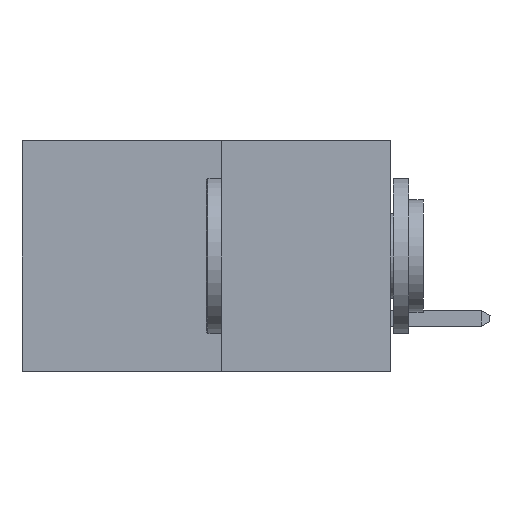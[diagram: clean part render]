
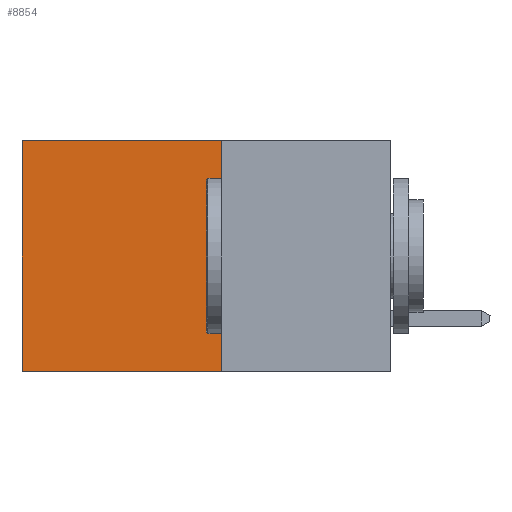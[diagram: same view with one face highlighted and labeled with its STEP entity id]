
A CAD part, left-side view. The second image highlights one B-rep face of the part: STEP entity #8854.
In plain terms, the highlighted planar face has unit normal (-1, 0, 0).
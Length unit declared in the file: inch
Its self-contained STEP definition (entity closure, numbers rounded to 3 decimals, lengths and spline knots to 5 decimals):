
#710 = ORIENTED_EDGE ( 'NONE', *, *, #8737, .F. ) ;
#855 = VERTEX_POINT ( 'NONE', #5815 ) ;
#1616 = LINE ( 'NONE', #2722, #4988 ) ;
#1722 = LINE ( 'NONE', #2775, #11220 ) ;
#2062 = DIRECTION ( 'NONE',  ( 0., 1., 0. ) ) ;
#2660 = CARTESIAN_POINT ( 'NONE',  ( 0.277, 0.27, -0.37 ) ) ;
#2722 = CARTESIAN_POINT ( 'NONE',  ( 0.277, 0.27, 0. ) ) ;
#2775 = CARTESIAN_POINT ( 'NONE',  ( 0.277, 0.59, -0.37 ) ) ;
#2887 = EDGE_CURVE ( 'NONE', #12410, #11856, #1616, .T. ) ;
#2941 = CARTESIAN_POINT ( 'NONE',  ( 0.277, 0.59, 0. ) ) ;
#2951 = ORIENTED_EDGE ( 'NONE', *, *, #4583, .F. ) ;
#3104 = FACE_OUTER_BOUND ( 'NONE', #4551, .T. ) ;
#3959 = DIRECTION ( 'NONE',  ( 0., 0., -1. ) ) ;
#4240 = PLANE ( 'NONE',  #6954 ) ;
#4551 = EDGE_LOOP ( 'NONE', ( #8530, #2951, #710, #6911 ) ) ;
#4583 = EDGE_CURVE ( 'NONE', #10110, #855, #14548, .T. ) ;
#4751 = VECTOR ( 'NONE', #6585, 39.37008 ) ;
#4988 = VECTOR ( 'NONE', #2062, 39.37008 ) ;
#5305 = DIRECTION ( 'NONE',  ( 0., 0., -1. ) ) ;
#5442 = CARTESIAN_POINT ( 'NONE',  ( 0.277, 0.27, -0.37 ) ) ;
#5647 = CARTESIAN_POINT ( 'NONE',  ( 0.277, 0.27, -0.37 ) ) ;
#5815 = CARTESIAN_POINT ( 'NONE',  ( 0.277, 0.59, -0.37 ) ) ;
#6567 = CARTESIAN_POINT ( 'NONE',  ( 0.277, 0.27, 0. ) ) ;
#6585 = DIRECTION ( 'NONE',  ( 0., 1., 0. ) ) ;
#6653 = CARTESIAN_POINT ( 'NONE',  ( 0.277, 0.27, -0.37 ) ) ;
#6911 = ORIENTED_EDGE ( 'NONE', *, *, #2887, .T. ) ;
#6954 = AXIS2_PLACEMENT_3D ( 'NONE', #6653, #14870, #7887 ) ;
#7887 = DIRECTION ( 'NONE',  ( 0., 0., -1. ) ) ;
#8530 = ORIENTED_EDGE ( 'NONE', *, *, #8776, .T. ) ;
#8737 = EDGE_CURVE ( 'NONE', #12410, #10110, #14831, .T. ) ;
#8776 = EDGE_CURVE ( 'NONE', #11856, #855, #1722, .T. ) ;
#8854 = ADVANCED_FACE ( 'NONE', ( #3104 ), #4240, .F. ) ;
#10110 = VERTEX_POINT ( 'NONE', #5647 ) ;
#11220 = VECTOR ( 'NONE', #5305, 39.37008 ) ;
#11856 = VERTEX_POINT ( 'NONE', #2941 ) ;
#11980 = VECTOR ( 'NONE', #3959, 39.37008 ) ;
#12410 = VERTEX_POINT ( 'NONE', #6567 ) ;
#14548 = LINE ( 'NONE', #5442, #4751 ) ;
#14831 = LINE ( 'NONE', #2660, #11980 ) ;
#14870 = DIRECTION ( 'NONE',  ( 1., 0., 0. ) ) ;
